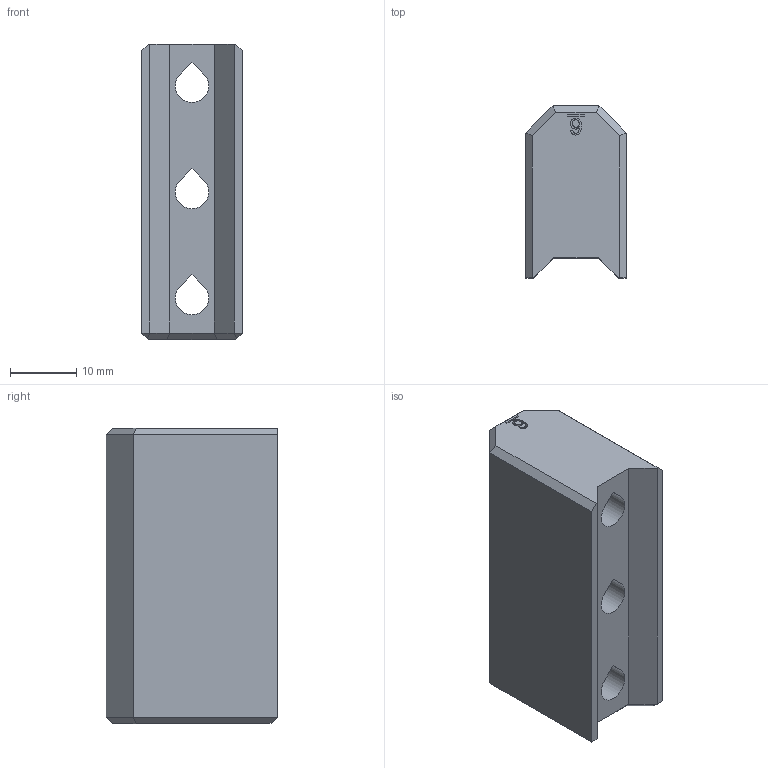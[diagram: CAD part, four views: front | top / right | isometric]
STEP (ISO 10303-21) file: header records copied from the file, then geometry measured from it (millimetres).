
FILE_DESCRIPTION(/* description */ (''),/* implementation_level */ '2;1');
FILE_NAME(/* name */ 'Riser 6 - 2.28.step',/* time_stamp */ '2023-02-26T21:26:00-06:00',/* author */ (''),/* organization */ (''),/* preprocessor_version */ 'ST-DEVELOPER v19.2',/* originating_system */ 'Autodesk Translation Framework v11.17.0.187',/* authorisation */ '');
FILE_SCHEMA (('AUTOMOTIVE_DESIGN { 1 0 10303 214 3 1 1 }'));
Length unit declared in the file: millimetre
Products named in the file (1): LPL Trijicon Mount (1.175")
Bounding box: 15.15 x 25.91 x 44.5 mm (x, y, z)
Volume: 13903.8 mm3; surface area: 5194.5 mm2
Topology: 1 solids, 1 shells, 71 faces, 184 edges, 118 vertices
Faces by surface type: plane 41, bspline 27, cylinder 3
Entity records: 2427 total; most frequent: CARTESIAN_POINT 833, ORIENTED_EDGE 368, DIRECTION 226, EDGE_CURVE 184, LINE 124, VECTOR 124, VERTEX_POINT 118, EDGE_LOOP 80
